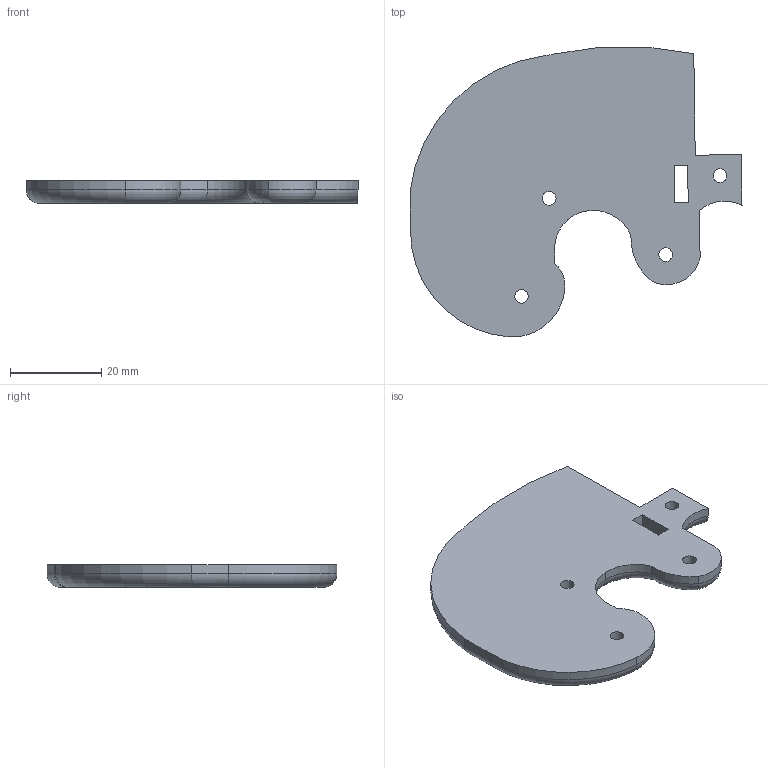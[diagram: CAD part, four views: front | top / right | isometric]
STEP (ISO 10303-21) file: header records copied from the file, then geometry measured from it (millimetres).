
FILE_DESCRIPTION((''),'2;1');
FILE_NAME('frame_R.stp','2013-08-15T20:11:37',('mrfr'),(''),'Autodesk Inventor 2013','Autodesk Inventor 2013','');
FILE_SCHEMA(('AUTOMOTIVE_DESIGN { 1 0 10303 214 1 1 1 1 }'));
Length unit declared in the file: millimetre
Products named in the file (1): frame_R
Bounding box: 72.68 x 63.45 x 5 mm (x, y, z)
Volume: 14208.7 mm3; surface area: 7605.4 mm2
Topology: 1 solids, 1 shells, 204 faces, 630 edges, 511 vertices
Faces by surface type: plane 146, bspline 26, cylinder 21, torus 11
Full cylindrical faces by diameter (mm): 3 x4
Entity records: 7503 total; most frequent: CARTESIAN_POINT 1759, ORIENTED_EDGE 1102, DIRECTION 1004, EDGE_CURVE 551, VECTOR 478, LINE 478, VERTEX_POINT 365, AXIS2_PLACEMENT_3D 263
